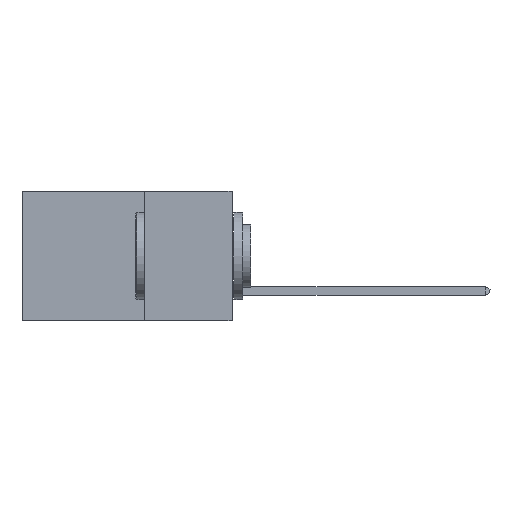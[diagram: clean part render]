
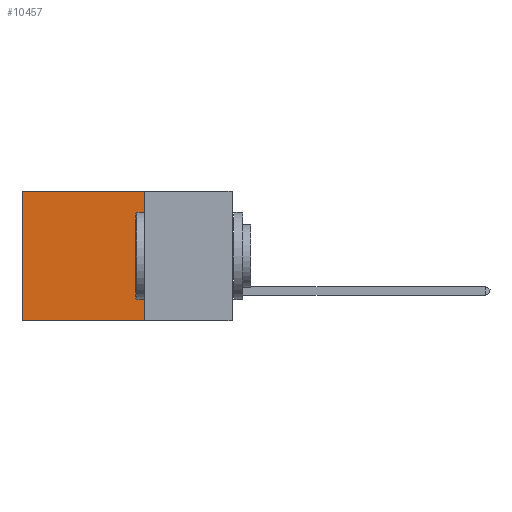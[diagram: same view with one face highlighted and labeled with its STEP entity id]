
A CAD part, left-side view. The second image highlights one B-rep face of the part: STEP entity #10457.
In plain terms, the highlighted planar face has unit normal (-1, 0, 0).
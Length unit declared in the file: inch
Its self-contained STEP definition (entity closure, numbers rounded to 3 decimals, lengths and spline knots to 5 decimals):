
#129 = EDGE_CURVE ( 'NONE', #7664, #12260, #16090, .T. ) ;
#437 = VECTOR ( 'NONE', #3508, 39.37008 ) ;
#1253 = CARTESIAN_POINT ( 'NONE',  ( 0.2875, 0.6, 0. ) ) ;
#1865 = CARTESIAN_POINT ( 'NONE',  ( 0.2875, 0.25, 0. ) ) ;
#3129 = ORIENTED_EDGE ( 'NONE', *, *, #5868, .F. ) ;
#3508 = DIRECTION ( 'NONE',  ( 0., 0., -1. ) ) ;
#3512 = VECTOR ( 'NONE', #13552, 39.37008 ) ;
#3957 = EDGE_CURVE ( 'NONE', #15252, #7664, #13356, .T. ) ;
#4438 = CARTESIAN_POINT ( 'NONE',  ( 0.2875, 0.25, -0.37 ) ) ;
#4726 = LINE ( 'NONE', #4438, #3512 ) ;
#5731 = DIRECTION ( 'NONE',  ( 1., 0., 0. ) ) ;
#5812 = EDGE_LOOP ( 'NONE', ( #14441, #3129, #10815, #9742 ) ) ;
#5868 = EDGE_CURVE ( 'NONE', #9609, #12260, #4726, .T. ) ;
#6561 = CARTESIAN_POINT ( 'NONE',  ( 0.2875, 0.6, -0.37 ) ) ;
#7295 = CARTESIAN_POINT ( 'NONE',  ( 0.2875, 0.25, 0. ) ) ;
#7664 = VERTEX_POINT ( 'NONE', #1253 ) ;
#8060 = CARTESIAN_POINT ( 'NONE',  ( 0.2875, 0.25, 0. ) ) ;
#9043 = PLANE ( 'NONE',  #13752 ) ;
#9066 = VECTOR ( 'NONE', #9224, 39.37008 ) ;
#9224 = DIRECTION ( 'NONE',  ( 0., 1., 0. ) ) ;
#9358 = CARTESIAN_POINT ( 'NONE',  ( 0.2875, 0.6, 0. ) ) ;
#9609 = VERTEX_POINT ( 'NONE', #13508 ) ;
#9742 = ORIENTED_EDGE ( 'NONE', *, *, #3957, .T. ) ;
#10457 = ADVANCED_FACE ( 'NONE', ( #12602 ), #9043, .F. ) ;
#10815 = ORIENTED_EDGE ( 'NONE', *, *, #15103, .F. ) ;
#11719 = DIRECTION ( 'NONE',  ( 0., 0., -1. ) ) ;
#12098 = CARTESIAN_POINT ( 'NONE',  ( 0.2875, 0.25, 0. ) ) ;
#12260 = VERTEX_POINT ( 'NONE', #6561 ) ;
#12602 = FACE_OUTER_BOUND ( 'NONE', #5812, .T. ) ;
#13356 = LINE ( 'NONE', #8060, #9066 ) ;
#13487 = LINE ( 'NONE', #7295, #437 ) ;
#13508 = CARTESIAN_POINT ( 'NONE',  ( 0.2875, 0.25, -0.37 ) ) ;
#13552 = DIRECTION ( 'NONE',  ( 0., 1., 0. ) ) ;
#13752 = AXIS2_PLACEMENT_3D ( 'NONE', #1865, #5731, #16204 ) ;
#14441 = ORIENTED_EDGE ( 'NONE', *, *, #129, .T. ) ;
#15103 = EDGE_CURVE ( 'NONE', #15252, #9609, #13487, .T. ) ;
#15252 = VERTEX_POINT ( 'NONE', #12098 ) ;
#15691 = VECTOR ( 'NONE', #11719, 39.37008 ) ;
#16090 = LINE ( 'NONE', #9358, #15691 ) ;
#16204 = DIRECTION ( 'NONE',  ( 0., 0., -1. ) ) ;
